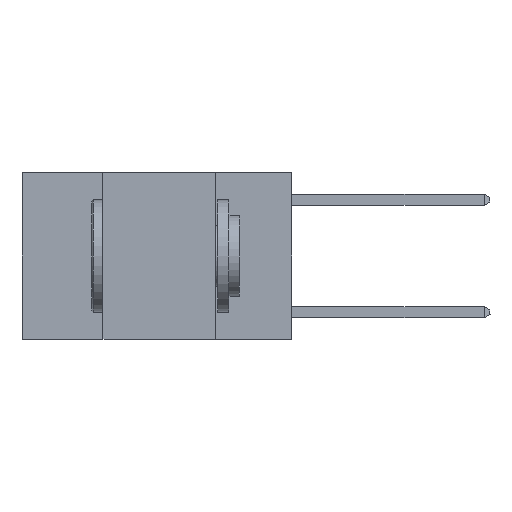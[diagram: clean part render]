
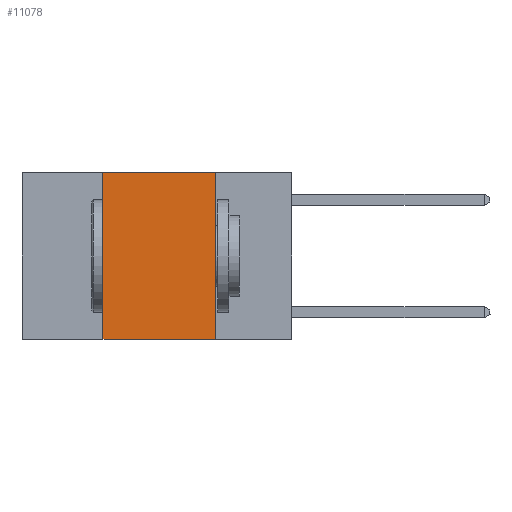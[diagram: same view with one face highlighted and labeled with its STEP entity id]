
A CAD part, left-side view. The second image highlights one B-rep face of the part: STEP entity #11078.
In plain terms, the highlighted planar face has unit normal (-1, 0, 0).
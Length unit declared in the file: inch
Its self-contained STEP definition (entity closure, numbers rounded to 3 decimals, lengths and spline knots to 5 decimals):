
#262 = CARTESIAN_POINT ( 'NONE',  ( 0., 0.6, 0. ) ) ;
#447 = LINE ( 'NONE', #2075, #6264 ) ;
#931 = LINE ( 'NONE', #262, #12787 ) ;
#1270 = CARTESIAN_POINT ( 'NONE',  ( 0., 0.17, 0. ) ) ;
#2075 = CARTESIAN_POINT ( 'NONE',  ( 0., 0.17, 0. ) ) ;
#2263 = ORIENTED_EDGE ( 'NONE', *, *, #7121, .F. ) ;
#3183 = DIRECTION ( 'NONE',  ( 0., 0., -1. ) ) ;
#4107 = EDGE_CURVE ( 'NONE', #14249, #11260, #931, .T. ) ;
#4409 = PLANE ( 'NONE',  #5539 ) ;
#4703 = DIRECTION ( 'NONE',  ( 0., -1., 0. ) ) ;
#5309 = VERTEX_POINT ( 'NONE', #11158 ) ;
#5539 = AXIS2_PLACEMENT_3D ( 'NONE', #6728, #6780, #14641 ) ;
#5577 = CARTESIAN_POINT ( 'NONE',  ( 0., 0.42, 0. ) ) ;
#5890 = LINE ( 'NONE', #9187, #10903 ) ;
#6264 = VECTOR ( 'NONE', #3183, 39.37008 ) ;
#6728 = CARTESIAN_POINT ( 'NONE',  ( 0., 0.6, 0. ) ) ;
#6780 = DIRECTION ( 'NONE',  ( 1., 0., 0. ) ) ;
#6809 = LINE ( 'NONE', #8198, #9493 ) ;
#7121 = EDGE_CURVE ( 'NONE', #11260, #9857, #447, .T. ) ;
#7194 = EDGE_CURVE ( 'NONE', #5309, #14249, #5890, .T. ) ;
#7266 = EDGE_CURVE ( 'NONE', #5309, #9857, #6809, .T. ) ;
#8198 = CARTESIAN_POINT ( 'NONE',  ( 0., 0.6, -0.37 ) ) ;
#8401 = DIRECTION ( 'NONE',  ( 0., -1., 0. ) ) ;
#8833 = ORIENTED_EDGE ( 'NONE', *, *, #7194, .F. ) ;
#9187 = CARTESIAN_POINT ( 'NONE',  ( 0., 0.42, 0. ) ) ;
#9493 = VECTOR ( 'NONE', #4703, 39.37008 ) ;
#9857 = VERTEX_POINT ( 'NONE', #13614 ) ;
#10300 = DIRECTION ( 'NONE',  ( 0., 0., 1. ) ) ;
#10903 = VECTOR ( 'NONE', #10300, 39.37008 ) ;
#11078 = ADVANCED_FACE ( 'NONE', ( #11424 ), #4409, .F. ) ;
#11158 = CARTESIAN_POINT ( 'NONE',  ( 0., 0.42, -0.37 ) ) ;
#11260 = VERTEX_POINT ( 'NONE', #1270 ) ;
#11424 = FACE_OUTER_BOUND ( 'NONE', #14263, .T. ) ;
#11811 = ORIENTED_EDGE ( 'NONE', *, *, #7266, .T. ) ;
#12787 = VECTOR ( 'NONE', #8401, 39.37008 ) ;
#13614 = CARTESIAN_POINT ( 'NONE',  ( 0., 0.17, -0.37 ) ) ;
#14249 = VERTEX_POINT ( 'NONE', #5577 ) ;
#14263 = EDGE_LOOP ( 'NONE', ( #2263, #14363, #8833, #11811 ) ) ;
#14363 = ORIENTED_EDGE ( 'NONE', *, *, #4107, .F. ) ;
#14641 = DIRECTION ( 'NONE',  ( 0., 0., -1. ) ) ;
